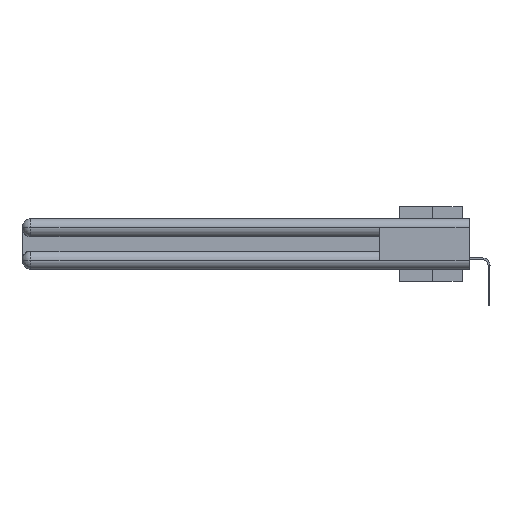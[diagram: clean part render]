
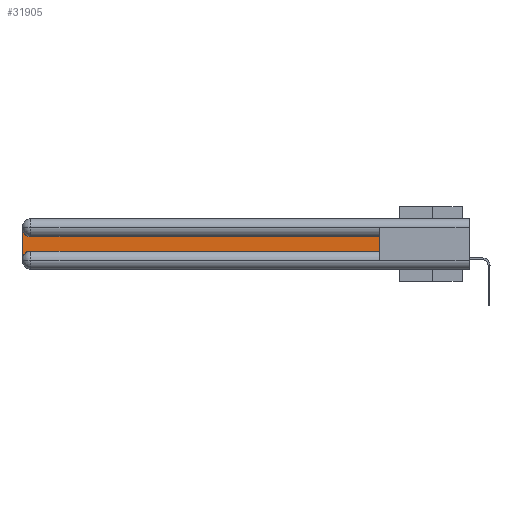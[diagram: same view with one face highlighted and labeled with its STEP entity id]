
A CAD part, left-side view. The second image highlights one B-rep face of the part: STEP entity #31905.
In plain terms, the highlighted planar face has unit normal (-1, 0, 0).
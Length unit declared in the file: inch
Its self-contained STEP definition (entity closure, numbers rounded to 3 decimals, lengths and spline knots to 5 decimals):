
#2179 = VECTOR ( 'NONE', #4959, 39.37008 ) ;
#2858 = VERTEX_POINT ( 'NONE', #34657 ) ;
#3052 = DIRECTION ( 'NONE',  ( 0., 0., -1. ) ) ;
#4328 = CIRCLE ( 'NONE', #36980, 0.06 ) ;
#4771 = VERTEX_POINT ( 'NONE', #27807 ) ;
#4881 = LINE ( 'NONE', #5014, #9054 ) ;
#4959 = DIRECTION ( 'NONE',  ( 0., 0., -1. ) ) ;
#5014 = CARTESIAN_POINT ( 'NONE',  ( 0.075, 0.6, -0.2175 ) ) ;
#5343 = DIRECTION ( 'NONE',  ( 0., 0., -1. ) ) ;
#5368 = VERTEX_POINT ( 'NONE', #10065 ) ;
#7299 = LINE ( 'NONE', #8598, #2179 ) ;
#8598 = CARTESIAN_POINT ( 'NONE',  ( 0.075, 3., -0.2175 ) ) ;
#9054 = VECTOR ( 'NONE', #31782, 39.37008 ) ;
#9623 = EDGE_CURVE ( 'NONE', #4771, #2858, #20166, .T. ) ;
#9902 = DIRECTION ( 'NONE',  ( 0., 1., 0. ) ) ;
#10065 = CARTESIAN_POINT ( 'NONE',  ( 0.075, 3., -0.2775 ) ) ;
#10220 = CIRCLE ( 'NONE', #19231, 0.06 ) ;
#12063 = VECTOR ( 'NONE', #14696, 39.37008 ) ;
#13082 = ORIENTED_EDGE ( 'NONE', *, *, #27300, .T. ) ;
#13709 = PLANE ( 'NONE',  #35012 ) ;
#13755 = VERTEX_POINT ( 'NONE', #23683 ) ;
#14696 = DIRECTION ( 'NONE',  ( 0., -1., 0. ) ) ;
#15156 = CARTESIAN_POINT ( 'NONE',  ( 0.075, 2.94, -0.0625 ) ) ;
#17189 = CARTESIAN_POINT ( 'NONE',  ( 0.075, 2.94, -0.2775 ) ) ;
#19177 = CARTESIAN_POINT ( 'NONE',  ( 0.075, 0.6, -0.1225 ) ) ;
#19231 = AXIS2_PLACEMENT_3D ( 'NONE', #15156, #32804, #3052 ) ;
#19870 = DIRECTION ( 'NONE',  ( 1., 0., 0. ) ) ;
#20166 = LINE ( 'NONE', #19177, #33208 ) ;
#20386 = FACE_OUTER_BOUND ( 'NONE', #24583, .T. ) ;
#21748 = VERTEX_POINT ( 'NONE', #22436 ) ;
#21834 = ORIENTED_EDGE ( 'NONE', *, *, #38181, .T. ) ;
#22436 = CARTESIAN_POINT ( 'NONE',  ( 0.075, 3., -0.0625 ) ) ;
#23193 = DIRECTION ( 'NONE',  ( 1., 0., 0. ) ) ;
#23492 = VERTEX_POINT ( 'NONE', #30560 ) ;
#23683 = CARTESIAN_POINT ( 'NONE',  ( 0.075, 2.94, -0.2175 ) ) ;
#24583 = EDGE_LOOP ( 'NONE', ( #33716, #32779, #13082, #21834, #26518, #24914 ) ) ;
#24682 = LINE ( 'NONE', #26432, #12063 ) ;
#24914 = ORIENTED_EDGE ( 'NONE', *, *, #33112, .T. ) ;
#26432 = CARTESIAN_POINT ( 'NONE',  ( 0.075, 0.6, -0.2175 ) ) ;
#26518 = ORIENTED_EDGE ( 'NONE', *, *, #30429, .T. ) ;
#27300 = EDGE_CURVE ( 'NONE', #21748, #5368, #7299, .T. ) ;
#27807 = CARTESIAN_POINT ( 'NONE',  ( 0.075, 0.6, -0.1225 ) ) ;
#28850 = CARTESIAN_POINT ( 'NONE',  ( 0.075, 3., -0.1225 ) ) ;
#30429 = EDGE_CURVE ( 'NONE', #13755, #23492, #24682, .T. ) ;
#30560 = CARTESIAN_POINT ( 'NONE',  ( 0.075, 0.6, -0.2175 ) ) ;
#31074 = EDGE_CURVE ( 'NONE', #2858, #21748, #10220, .T. ) ;
#31747 = DIRECTION ( 'NONE',  ( 0., 0., -1. ) ) ;
#31782 = DIRECTION ( 'NONE',  ( 0., 0., 1. ) ) ;
#31905 = ADVANCED_FACE ( 'NONE', ( #20386 ), #13709, .F. ) ;
#32779 = ORIENTED_EDGE ( 'NONE', *, *, #31074, .T. ) ;
#32804 = DIRECTION ( 'NONE',  ( 1., 0., 0. ) ) ;
#33112 = EDGE_CURVE ( 'NONE', #23492, #4771, #4881, .T. ) ;
#33208 = VECTOR ( 'NONE', #9902, 39.37008 ) ;
#33716 = ORIENTED_EDGE ( 'NONE', *, *, #9623, .T. ) ;
#34657 = CARTESIAN_POINT ( 'NONE',  ( 0.075, 2.94, -0.1225 ) ) ;
#35012 = AXIS2_PLACEMENT_3D ( 'NONE', #28850, #19870, #31747 ) ;
#36980 = AXIS2_PLACEMENT_3D ( 'NONE', #17189, #23193, #5343 ) ;
#38181 = EDGE_CURVE ( 'NONE', #5368, #13755, #4328, .T. ) ;
